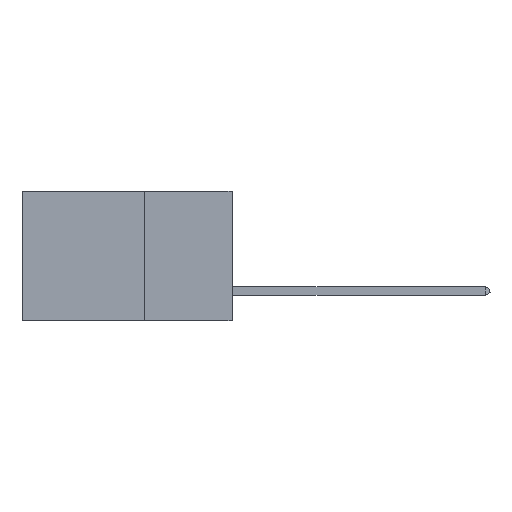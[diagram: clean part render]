
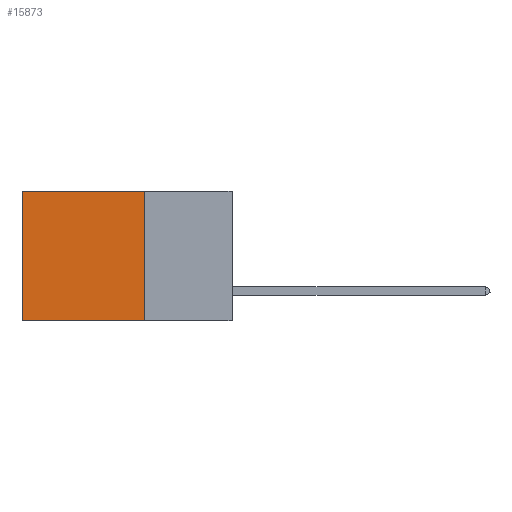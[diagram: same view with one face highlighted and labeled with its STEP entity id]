
A CAD part, left-side view. The second image highlights one B-rep face of the part: STEP entity #15873.
In plain terms, the highlighted planar face has unit normal (-1, 0, 0).
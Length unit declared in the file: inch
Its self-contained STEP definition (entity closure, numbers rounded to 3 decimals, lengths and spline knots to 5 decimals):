
#6 = EDGE_CURVE ( 'NONE', #584, #2202, #9076, .T. ) ;
#110 = VECTOR ( 'NONE', #17297, 39.37008 ) ;
#331 = DIRECTION ( 'NONE',  ( 1., 0., 0. ) ) ;
#567 = LINE ( 'NONE', #12745, #8029 ) ;
#584 = VERTEX_POINT ( 'NONE', #22155 ) ;
#1897 = CARTESIAN_POINT ( 'NONE',  ( 0.2875, 0.6, 0. ) ) ;
#2202 = VERTEX_POINT ( 'NONE', #14922 ) ;
#3959 = CARTESIAN_POINT ( 'NONE',  ( 0.2875, 0.25, -0.37 ) ) ;
#5447 = DIRECTION ( 'NONE',  ( 0., 1., 0. ) ) ;
#5738 = CARTESIAN_POINT ( 'NONE',  ( 0.2875, 0.25, 0. ) ) ;
#6219 = VERTEX_POINT ( 'NONE', #20867 ) ;
#6729 = LINE ( 'NONE', #22450, #11162 ) ;
#8029 = VECTOR ( 'NONE', #16464, 39.37008 ) ;
#8100 = EDGE_LOOP ( 'NONE', ( #8274, #14228, #17469, #19674 ) ) ;
#8274 = ORIENTED_EDGE ( 'NONE', *, *, #16316, .T. ) ;
#9076 = LINE ( 'NONE', #3959, #18772 ) ;
#10966 = VERTEX_POINT ( 'NONE', #1897 ) ;
#11162 = VECTOR ( 'NONE', #5447, 39.37008 ) ;
#11413 = EDGE_CURVE ( 'NONE', #6219, #584, #13717, .T. ) ;
#11929 = EDGE_CURVE ( 'NONE', #6219, #10966, #6729, .T. ) ;
#12745 = CARTESIAN_POINT ( 'NONE',  ( 0.2875, 0.6, 0. ) ) ;
#13717 = LINE ( 'NONE', #22863, #110 ) ;
#14228 = ORIENTED_EDGE ( 'NONE', *, *, #6, .F. ) ;
#14370 = DIRECTION ( 'NONE',  ( 0., 0., -1. ) ) ;
#14522 = DIRECTION ( 'NONE',  ( 0., 1., 0. ) ) ;
#14922 = CARTESIAN_POINT ( 'NONE',  ( 0.2875, 0.6, -0.37 ) ) ;
#15551 = AXIS2_PLACEMENT_3D ( 'NONE', #5738, #331, #14370 ) ;
#15873 = ADVANCED_FACE ( 'NONE', ( #17214 ), #16366, .F. ) ;
#16316 = EDGE_CURVE ( 'NONE', #10966, #2202, #567, .T. ) ;
#16366 = PLANE ( 'NONE',  #15551 ) ;
#16464 = DIRECTION ( 'NONE',  ( 0., 0., -1. ) ) ;
#17214 = FACE_OUTER_BOUND ( 'NONE', #8100, .T. ) ;
#17297 = DIRECTION ( 'NONE',  ( 0., 0., -1. ) ) ;
#17469 = ORIENTED_EDGE ( 'NONE', *, *, #11413, .F. ) ;
#18772 = VECTOR ( 'NONE', #14522, 39.37008 ) ;
#19674 = ORIENTED_EDGE ( 'NONE', *, *, #11929, .T. ) ;
#20867 = CARTESIAN_POINT ( 'NONE',  ( 0.2875, 0.25, 0. ) ) ;
#22155 = CARTESIAN_POINT ( 'NONE',  ( 0.2875, 0.25, -0.37 ) ) ;
#22450 = CARTESIAN_POINT ( 'NONE',  ( 0.2875, 0.25, 0. ) ) ;
#22863 = CARTESIAN_POINT ( 'NONE',  ( 0.2875, 0.25, 0. ) ) ;
